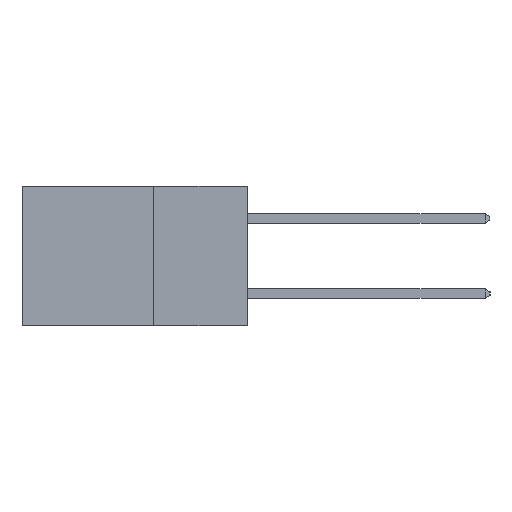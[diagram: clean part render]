
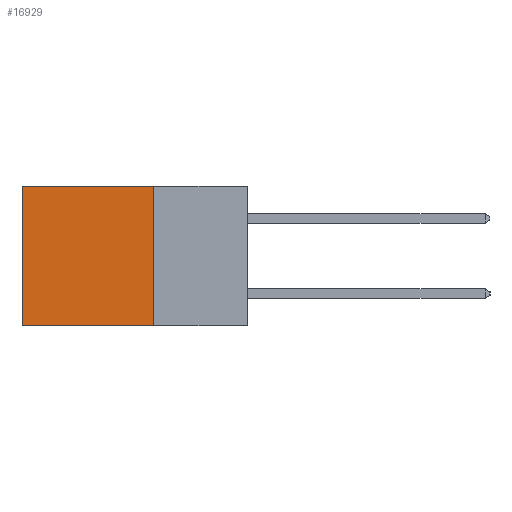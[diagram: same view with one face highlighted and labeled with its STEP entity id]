
A CAD part, left-side view. The second image highlights one B-rep face of the part: STEP entity #16929.
In plain terms, the highlighted planar face has unit normal (-1, 0, 0).
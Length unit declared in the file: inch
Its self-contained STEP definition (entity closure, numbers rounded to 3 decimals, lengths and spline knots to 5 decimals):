
#218 = ORIENTED_EDGE ( 'NONE', *, *, #9083, .T. ) ;
#438 = DIRECTION ( 'NONE',  ( 0., 1., 0. ) ) ;
#722 = CARTESIAN_POINT ( 'NONE',  ( 0.2615, 0.25, 0. ) ) ;
#1357 = VECTOR ( 'NONE', #14955, 39.37008 ) ;
#2560 = VERTEX_POINT ( 'NONE', #14275 ) ;
#2595 = CARTESIAN_POINT ( 'NONE',  ( 0.2615, 0.6, -0.37 ) ) ;
#2653 = CARTESIAN_POINT ( 'NONE',  ( 0.2615, 0.6, 0. ) ) ;
#3277 = EDGE_LOOP ( 'NONE', ( #18408, #16464, #13460, #218 ) ) ;
#4315 = LINE ( 'NONE', #8920, #8304 ) ;
#4431 = DIRECTION ( 'NONE',  ( 0., 0., -1. ) ) ;
#4434 = FACE_OUTER_BOUND ( 'NONE', #3277, .T. ) ;
#5899 = DIRECTION ( 'NONE',  ( 0., 1., 0. ) ) ;
#6397 = VECTOR ( 'NONE', #5899, 39.37008 ) ;
#6663 = CARTESIAN_POINT ( 'NONE',  ( 0.2615, 0.25, -0.37 ) ) ;
#6679 = LINE ( 'NONE', #2595, #14943 ) ;
#7692 = DIRECTION ( 'NONE',  ( 0., 0., -1. ) ) ;
#7770 = CARTESIAN_POINT ( 'NONE',  ( 0.2615, 0.25, -0.37 ) ) ;
#8304 = VECTOR ( 'NONE', #438, 39.37008 ) ;
#8412 = EDGE_CURVE ( 'NONE', #12121, #13979, #6679, .T. ) ;
#8920 = CARTESIAN_POINT ( 'NONE',  ( 0.2615, 0.25, -0.37 ) ) ;
#9083 = EDGE_CURVE ( 'NONE', #10225, #12121, #15175, .T. ) ;
#10225 = VERTEX_POINT ( 'NONE', #18770 ) ;
#12121 = VERTEX_POINT ( 'NONE', #2653 ) ;
#13460 = ORIENTED_EDGE ( 'NONE', *, *, #14450, .F. ) ;
#13536 = CARTESIAN_POINT ( 'NONE',  ( 0.2615, 0.6, -0.37 ) ) ;
#13979 = VERTEX_POINT ( 'NONE', #13536 ) ;
#14106 = EDGE_CURVE ( 'NONE', #2560, #13979, #4315, .T. ) ;
#14275 = CARTESIAN_POINT ( 'NONE',  ( 0.2615, 0.25, -0.37 ) ) ;
#14399 = DIRECTION ( 'NONE',  ( 1., 0., 0. ) ) ;
#14450 = EDGE_CURVE ( 'NONE', #10225, #2560, #14732, .T. ) ;
#14732 = LINE ( 'NONE', #6663, #1357 ) ;
#14943 = VECTOR ( 'NONE', #7692, 39.37008 ) ;
#14955 = DIRECTION ( 'NONE',  ( 0., 0., -1. ) ) ;
#15175 = LINE ( 'NONE', #722, #6397 ) ;
#16433 = AXIS2_PLACEMENT_3D ( 'NONE', #7770, #14399, #4431 ) ;
#16464 = ORIENTED_EDGE ( 'NONE', *, *, #14106, .F. ) ;
#16929 = ADVANCED_FACE ( 'NONE', ( #4434 ), #19191, .F. ) ;
#18408 = ORIENTED_EDGE ( 'NONE', *, *, #8412, .T. ) ;
#18770 = CARTESIAN_POINT ( 'NONE',  ( 0.2615, 0.25, 0. ) ) ;
#19191 = PLANE ( 'NONE',  #16433 ) ;
